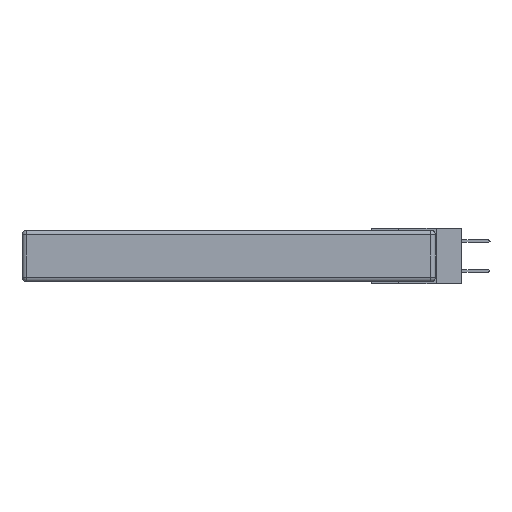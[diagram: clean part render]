
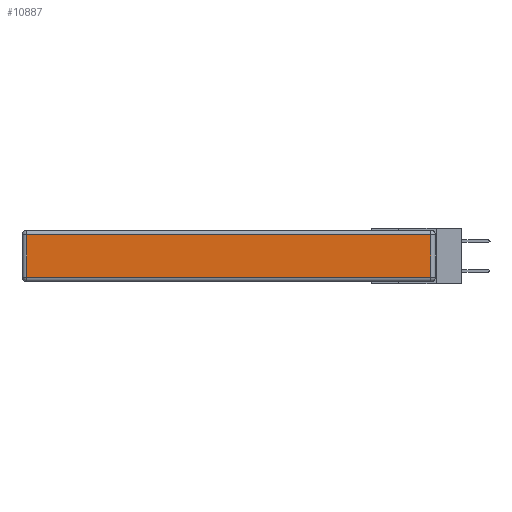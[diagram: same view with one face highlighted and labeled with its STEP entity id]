
A CAD part, left-side view. The second image highlights one B-rep face of the part: STEP entity #10887.
In plain terms, the highlighted planar face has unit normal (-1, 0, 0).
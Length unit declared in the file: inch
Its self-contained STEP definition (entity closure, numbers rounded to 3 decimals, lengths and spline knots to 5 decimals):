
#2193 = VECTOR ( 'NONE', #26324, 39.37008 ) ;
#3304 = VERTEX_POINT ( 'NONE', #21355 ) ;
#4181 = DIRECTION ( 'NONE',  ( -1., 0., 0. ) ) ;
#4570 = LINE ( 'NONE', #13874, #19092 ) ;
#6928 = VERTEX_POINT ( 'NONE', #8881 ) ;
#7108 = VECTOR ( 'NONE', #20268, 39.37008 ) ;
#7850 = CARTESIAN_POINT ( 'NONE',  ( 0., 0.03, -0.313 ) ) ;
#8524 = DIRECTION ( 'NONE',  ( 0., 1., 0. ) ) ;
#8881 = CARTESIAN_POINT ( 'NONE',  ( 0., 0.03, -0.03 ) ) ;
#9019 = EDGE_CURVE ( 'NONE', #19868, #6928, #32381, .T. ) ;
#9822 = EDGE_CURVE ( 'NONE', #3304, #10307, #31447, .T. ) ;
#9915 = DIRECTION ( 'NONE',  ( 0., 0., -1. ) ) ;
#10307 = VERTEX_POINT ( 'NONE', #18506 ) ;
#10887 = ADVANCED_FACE ( 'NONE', ( #19026 ), #31098, .T. ) ;
#12416 = CARTESIAN_POINT ( 'NONE',  ( 0., 0., -0.343 ) ) ;
#12705 = CARTESIAN_POINT ( 'NONE',  ( 0., 2.72, -0.343 ) ) ;
#12730 = ORIENTED_EDGE ( 'NONE', *, *, #25895, .T. ) ;
#13874 = CARTESIAN_POINT ( 'NONE',  ( 0., 2.75, -0.03 ) ) ;
#14177 = EDGE_LOOP ( 'NONE', ( #21412, #31226, #12730, #29752 ) ) ;
#18506 = CARTESIAN_POINT ( 'NONE',  ( 0., 2.72, -0.313 ) ) ;
#19026 = FACE_OUTER_BOUND ( 'NONE', #14177, .T. ) ;
#19092 = VECTOR ( 'NONE', #8524, 39.37008 ) ;
#19868 = VERTEX_POINT ( 'NONE', #7850 ) ;
#20268 = DIRECTION ( 'NONE',  ( 0., 0., 1. ) ) ;
#20503 = DIRECTION ( 'NONE',  ( 0., 0., 1. ) ) ;
#20529 = EDGE_CURVE ( 'NONE', #10307, #19868, #32490, .T. ) ;
#21355 = CARTESIAN_POINT ( 'NONE',  ( 0., 2.72, -0.03 ) ) ;
#21412 = ORIENTED_EDGE ( 'NONE', *, *, #20529, .T. ) ;
#25895 = EDGE_CURVE ( 'NONE', #6928, #3304, #4570, .T. ) ;
#26324 = DIRECTION ( 'NONE',  ( 0., -1., 0. ) ) ;
#26784 = AXIS2_PLACEMENT_3D ( 'NONE', #12416, #4181, #20503 ) ;
#28058 = CARTESIAN_POINT ( 'NONE',  ( 0., 0.03, -0.343 ) ) ;
#28599 = CARTESIAN_POINT ( 'NONE',  ( 0., 0., -0.313 ) ) ;
#29752 = ORIENTED_EDGE ( 'NONE', *, *, #9822, .T. ) ;
#31098 = PLANE ( 'NONE',  #26784 ) ;
#31226 = ORIENTED_EDGE ( 'NONE', *, *, #9019, .T. ) ;
#31447 = LINE ( 'NONE', #12705, #31894 ) ;
#31894 = VECTOR ( 'NONE', #9915, 39.37008 ) ;
#32381 = LINE ( 'NONE', #28058, #7108 ) ;
#32490 = LINE ( 'NONE', #28599, #2193 ) ;
